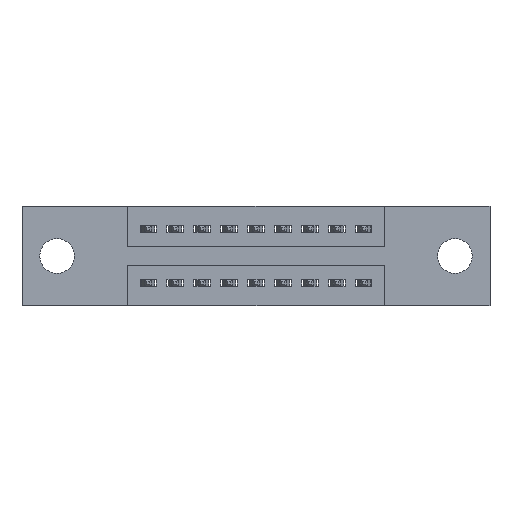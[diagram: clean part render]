
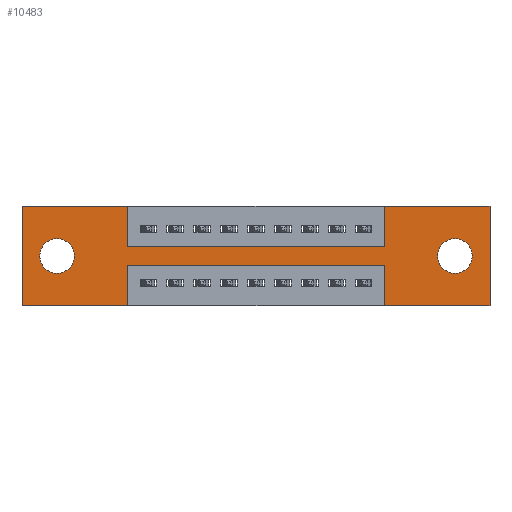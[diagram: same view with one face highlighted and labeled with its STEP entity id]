
A CAD part, front view. The second image highlights one B-rep face of the part: STEP entity #10483.
In plain terms, the highlighted planar face has unit normal (0, -1, 0).
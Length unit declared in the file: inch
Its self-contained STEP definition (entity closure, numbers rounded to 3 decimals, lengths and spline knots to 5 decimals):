
#52 = VECTOR ( 'NONE', #7712, 39.37008 ) ;
#106 = VECTOR ( 'NONE', #7866, 39.37008 ) ;
#120 = CARTESIAN_POINT ( 'NONE',  ( 0., 0., 0. ) ) ;
#178 = DIRECTION ( 'NONE',  ( 1., 0., 0. ) ) ;
#208 = VECTOR ( 'NONE', #178, 39.37008 ) ;
#249 = EDGE_CURVE ( 'NONE', #3354, #2344, #3117, .T. ) ;
#280 = LINE ( 'NONE', #2439, #2414 ) ;
#326 = CARTESIAN_POINT ( 'NONE',  ( 1.605, 0., -0.249 ) ) ;
#469 = CARTESIAN_POINT ( 'NONE',  ( 1.735, 0., 0. ) ) ;
#701 = EDGE_CURVE ( 'NONE', #788, #3045, #1131, .T. ) ;
#788 = VERTEX_POINT ( 'NONE', #6494 ) ;
#1010 = ORIENTED_EDGE ( 'NONE', *, *, #6233, .F. ) ;
#1130 = EDGE_CURVE ( 'NONE', #5972, #5124, #5488, .T. ) ;
#1131 = LINE ( 'NONE', #6876, #2094 ) ;
#1295 = ORIENTED_EDGE ( 'NONE', *, *, #3366, .F. ) ;
#1510 = CARTESIAN_POINT ( 'NONE',  ( 0.13, 0., -0.121 ) ) ;
#1519 = VERTEX_POINT ( 'NONE', #3665 ) ;
#1574 = ORIENTED_EDGE ( 'NONE', *, *, #2550, .F. ) ;
#1847 = ORIENTED_EDGE ( 'NONE', *, *, #3772, .F. ) ;
#1894 = CARTESIAN_POINT ( 'NONE',  ( 0., 0., -0.37 ) ) ;
#2027 = LINE ( 'NONE', #7932, #11242 ) ;
#2094 = VECTOR ( 'NONE', #8690, 39.37008 ) ;
#2150 = DIRECTION ( 'NONE',  ( 0., 0., -1. ) ) ;
#2193 = EDGE_CURVE ( 'NONE', #3045, #5816, #5751, .T. ) ;
#2205 = DIRECTION ( 'NONE',  ( 0., 1., 0. ) ) ;
#2332 = CARTESIAN_POINT ( 'NONE',  ( 1.605, 0., -0.185 ) ) ;
#2344 = VERTEX_POINT ( 'NONE', #8656 ) ;
#2413 = DIRECTION ( 'NONE',  ( 0., 0., 1. ) ) ;
#2414 = VECTOR ( 'NONE', #2413, 39.37008 ) ;
#2420 = VECTOR ( 'NONE', #5554, 39.37008 ) ;
#2439 = CARTESIAN_POINT ( 'NONE',  ( 0., 0., 0. ) ) ;
#2537 = LINE ( 'NONE', #7279, #106 ) ;
#2550 = EDGE_CURVE ( 'NONE', #9293, #7934, #9716, .T. ) ;
#2551 = ORIENTED_EDGE ( 'NONE', *, *, #701, .F. ) ;
#2580 = FACE_BOUND ( 'NONE', #5393, .T. ) ;
#2709 = LINE ( 'NONE', #9067, #2420 ) ;
#2927 = VECTOR ( 'NONE', #9303, 39.37008 ) ;
#2951 = VECTOR ( 'NONE', #8225, 39.37008 ) ;
#3017 = CARTESIAN_POINT ( 'NONE',  ( 1.3425, 0., -0.15 ) ) ;
#3045 = VERTEX_POINT ( 'NONE', #3908 ) ;
#3117 = CIRCLE ( 'NONE', #8236, 0.064 ) ;
#3273 = ORIENTED_EDGE ( 'NONE', *, *, #6502, .T. ) ;
#3316 = VECTOR ( 'NONE', #8448, 39.37008 ) ;
#3354 = VERTEX_POINT ( 'NONE', #326 ) ;
#3366 = EDGE_CURVE ( 'NONE', #8319, #4500, #7847, .T. ) ;
#3428 = ORIENTED_EDGE ( 'NONE', *, *, #9289, .F. ) ;
#3479 = AXIS2_PLACEMENT_3D ( 'NONE', #4769, #4725, #4676 ) ;
#3665 = CARTESIAN_POINT ( 'NONE',  ( 0.3925, 0., 0. ) ) ;
#3723 = ORIENTED_EDGE ( 'NONE', *, *, #9832, .F. ) ;
#3772 = EDGE_CURVE ( 'NONE', #7959, #1519, #5567, .T. ) ;
#3787 = VECTOR ( 'NONE', #4631, 39.37008 ) ;
#3860 = LINE ( 'NONE', #5242, #6398 ) ;
#3908 = CARTESIAN_POINT ( 'NONE',  ( 0.3925, 0., -0.37 ) ) ;
#4300 = DIRECTION ( 'NONE',  ( 0., 0., 1. ) ) ;
#4500 = VERTEX_POINT ( 'NONE', #469 ) ;
#4624 = ORIENTED_EDGE ( 'NONE', *, *, #2193, .F. ) ;
#4631 = DIRECTION ( 'NONE',  ( 0., 0., -1. ) ) ;
#4645 = CARTESIAN_POINT ( 'NONE',  ( 0.13, 0., -0.185 ) ) ;
#4676 = DIRECTION ( 'NONE',  ( 0., 0., 1. ) ) ;
#4720 = DIRECTION ( 'NONE',  ( 0., -1., 0. ) ) ;
#4725 = DIRECTION ( 'NONE',  ( 0., 1., 0. ) ) ;
#4769 = CARTESIAN_POINT ( 'NONE',  ( 0.13, 0., -0.185 ) ) ;
#4910 = CARTESIAN_POINT ( 'NONE',  ( 1.3425, 0., 0. ) ) ;
#5124 = VERTEX_POINT ( 'NONE', #6741 ) ;
#5242 = CARTESIAN_POINT ( 'NONE',  ( 0., 0., -0.37 ) ) ;
#5295 = EDGE_CURVE ( 'NONE', #10295, #10880, #10963, .T. ) ;
#5360 = CIRCLE ( 'NONE', #10253, 0.064 ) ;
#5393 = EDGE_LOOP ( 'NONE', ( #10695, #8982 ) ) ;
#5447 = EDGE_CURVE ( 'NONE', #5816, #7959, #280, .T. ) ;
#5488 = LINE ( 'NONE', #8333, #2951 ) ;
#5554 = DIRECTION ( 'NONE',  ( 0., 0., -1. ) ) ;
#5567 = LINE ( 'NONE', #8498, #3316 ) ;
#5751 = LINE ( 'NONE', #9257, #2927 ) ;
#5816 = VERTEX_POINT ( 'NONE', #9377 ) ;
#5934 = CIRCLE ( 'NONE', #6373, 0.064 ) ;
#5972 = VERTEX_POINT ( 'NONE', #9213 ) ;
#6013 = VERTEX_POINT ( 'NONE', #8280 ) ;
#6101 = EDGE_CURVE ( 'NONE', #10880, #10295, #5360, .T. ) ;
#6115 = ORIENTED_EDGE ( 'NONE', *, *, #249, .T. ) ;
#6140 = EDGE_CURVE ( 'NONE', #5124, #788, #2537, .T. ) ;
#6233 = EDGE_CURVE ( 'NONE', #6013, #5972, #3860, .T. ) ;
#6335 = LINE ( 'NONE', #8243, #3787 ) ;
#6373 = AXIS2_PLACEMENT_3D ( 'NONE', #10631, #10841, #9649 ) ;
#6398 = VECTOR ( 'NONE', #9673, 39.37008 ) ;
#6494 = CARTESIAN_POINT ( 'NONE',  ( 0.3925, 0., -0.22 ) ) ;
#6502 = EDGE_CURVE ( 'NONE', #2344, #3354, #5934, .T. ) ;
#6563 = ORIENTED_EDGE ( 'NONE', *, *, #11146, .F. ) ;
#6741 = CARTESIAN_POINT ( 'NONE',  ( 1.3425, 0., -0.22 ) ) ;
#6876 = CARTESIAN_POINT ( 'NONE',  ( 0.3925, 0., -0.37 ) ) ;
#6921 = DIRECTION ( 'NONE',  ( 0., 0., 1. ) ) ;
#7279 = CARTESIAN_POINT ( 'NONE',  ( 0.3925, 0., -0.22 ) ) ;
#7285 = FACE_BOUND ( 'NONE', #11471, .T. ) ;
#7508 = EDGE_LOOP ( 'NONE', ( #2551, #9782, #10305, #1010, #3428, #1295, #3723, #1574, #6563, #1847, #11316, #4624 ) ) ;
#7593 = CARTESIAN_POINT ( 'NONE',  ( 0.3925, 0., -0.15 ) ) ;
#7712 = DIRECTION ( 'NONE',  ( 1., 0., 0. ) ) ;
#7847 = LINE ( 'NONE', #120, #208 ) ;
#7866 = DIRECTION ( 'NONE',  ( -1., 0., 0. ) ) ;
#7932 = CARTESIAN_POINT ( 'NONE',  ( 1.3425, 0., 0. ) ) ;
#7934 = VERTEX_POINT ( 'NONE', #3017 ) ;
#7959 = VERTEX_POINT ( 'NONE', #8557 ) ;
#8225 = DIRECTION ( 'NONE',  ( 0., 0., 1. ) ) ;
#8236 = AXIS2_PLACEMENT_3D ( 'NONE', #2332, #2205, #2150 ) ;
#8243 = CARTESIAN_POINT ( 'NONE',  ( 1.735, 0., 0. ) ) ;
#8280 = CARTESIAN_POINT ( 'NONE',  ( 1.735, 0., -0.37 ) ) ;
#8319 = VERTEX_POINT ( 'NONE', #4910 ) ;
#8333 = CARTESIAN_POINT ( 'NONE',  ( 1.3425, 0., -0.37 ) ) ;
#8448 = DIRECTION ( 'NONE',  ( 1., 0., 0. ) ) ;
#8498 = CARTESIAN_POINT ( 'NONE',  ( 0., 0., 0. ) ) ;
#8557 = CARTESIAN_POINT ( 'NONE',  ( 0., 0., 0. ) ) ;
#8656 = CARTESIAN_POINT ( 'NONE',  ( 1.605, 0., -0.121 ) ) ;
#8690 = DIRECTION ( 'NONE',  ( 0., 0., -1. ) ) ;
#8982 = ORIENTED_EDGE ( 'NONE', *, *, #5295, .T. ) ;
#9067 = CARTESIAN_POINT ( 'NONE',  ( 0.3925, 0., 0. ) ) ;
#9213 = CARTESIAN_POINT ( 'NONE',  ( 1.3425, 0., -0.37 ) ) ;
#9257 = CARTESIAN_POINT ( 'NONE',  ( 0., 0., -0.37 ) ) ;
#9289 = EDGE_CURVE ( 'NONE', #4500, #6013, #6335, .T. ) ;
#9293 = VERTEX_POINT ( 'NONE', #9961 ) ;
#9303 = DIRECTION ( 'NONE',  ( -1., 0., 0. ) ) ;
#9377 = CARTESIAN_POINT ( 'NONE',  ( 0., 0., -0.37 ) ) ;
#9649 = DIRECTION ( 'NONE',  ( 0., 0., -1. ) ) ;
#9673 = DIRECTION ( 'NONE',  ( -1., 0., 0. ) ) ;
#9674 = CARTESIAN_POINT ( 'NONE',  ( 0.13, 0., -0.249 ) ) ;
#9716 = LINE ( 'NONE', #7593, #52 ) ;
#9782 = ORIENTED_EDGE ( 'NONE', *, *, #6140, .F. ) ;
#9805 = FACE_OUTER_BOUND ( 'NONE', #7508, .T. ) ;
#9832 = EDGE_CURVE ( 'NONE', #7934, #8319, #2027, .T. ) ;
#9896 = DIRECTION ( 'NONE',  ( 0., 1., 0. ) ) ;
#9961 = CARTESIAN_POINT ( 'NONE',  ( 0.3925, 0., -0.15 ) ) ;
#10042 = PLANE ( 'NONE',  #10116 ) ;
#10116 = AXIS2_PLACEMENT_3D ( 'NONE', #1894, #4720, #10874 ) ;
#10253 = AXIS2_PLACEMENT_3D ( 'NONE', #4645, #9896, #6921 ) ;
#10295 = VERTEX_POINT ( 'NONE', #9674 ) ;
#10305 = ORIENTED_EDGE ( 'NONE', *, *, #1130, .F. ) ;
#10483 = ADVANCED_FACE ( 'NONE', ( #7285, #2580, #9805 ), #10042, .T. ) ;
#10631 = CARTESIAN_POINT ( 'NONE',  ( 1.605, 0., -0.185 ) ) ;
#10695 = ORIENTED_EDGE ( 'NONE', *, *, #6101, .T. ) ;
#10841 = DIRECTION ( 'NONE',  ( 0., 1., 0. ) ) ;
#10874 = DIRECTION ( 'NONE',  ( 0., 0., -1. ) ) ;
#10880 = VERTEX_POINT ( 'NONE', #1510 ) ;
#10963 = CIRCLE ( 'NONE', #3479, 0.064 ) ;
#11146 = EDGE_CURVE ( 'NONE', #1519, #9293, #2709, .T. ) ;
#11242 = VECTOR ( 'NONE', #4300, 39.37008 ) ;
#11316 = ORIENTED_EDGE ( 'NONE', *, *, #5447, .F. ) ;
#11471 = EDGE_LOOP ( 'NONE', ( #3273, #6115 ) ) ;
